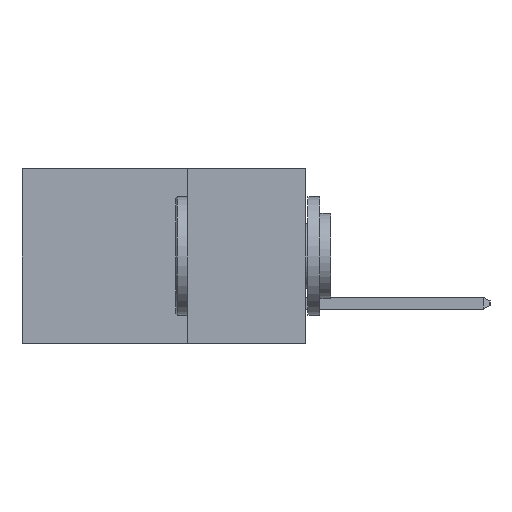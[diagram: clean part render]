
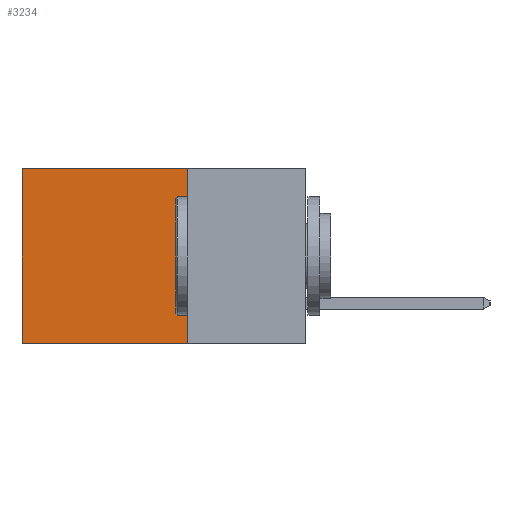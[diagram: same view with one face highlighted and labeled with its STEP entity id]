
A CAD part, left-side view. The second image highlights one B-rep face of the part: STEP entity #3234.
In plain terms, the highlighted planar face has unit normal (-1, 0, 0).
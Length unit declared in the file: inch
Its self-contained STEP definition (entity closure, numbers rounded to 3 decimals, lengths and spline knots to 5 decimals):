
#453 = VECTOR ( 'NONE', #2113, 39.37008 ) ;
#624 = CARTESIAN_POINT ( 'NONE',  ( 0.2615, 0.6, -0.37 ) ) ;
#630 = CARTESIAN_POINT ( 'NONE',  ( 0.2615, 0.25, 0. ) ) ;
#774 = CARTESIAN_POINT ( 'NONE',  ( 0.2615, 0.25, -0.37 ) ) ;
#1173 = EDGE_LOOP ( 'NONE', ( #9363, #12751, #15574, #9798 ) ) ;
#2059 = CARTESIAN_POINT ( 'NONE',  ( 0.2615, 0.25, -0.37 ) ) ;
#2113 = DIRECTION ( 'NONE',  ( 0., 0., -1. ) ) ;
#2167 = AXIS2_PLACEMENT_3D ( 'NONE', #13113, #12889, #12871 ) ;
#3066 = CARTESIAN_POINT ( 'NONE',  ( 0.2615, 0.25, -0.37 ) ) ;
#3168 = CARTESIAN_POINT ( 'NONE',  ( 0.2615, 0.6, 0. ) ) ;
#3234 = ADVANCED_FACE ( 'NONE', ( #12337 ), #14115, .F. ) ;
#3305 = DIRECTION ( 'NONE',  ( 0., 1., 0. ) ) ;
#3522 = VERTEX_POINT ( 'NONE', #3168 ) ;
#4558 = LINE ( 'NONE', #9187, #10623 ) ;
#4650 = VECTOR ( 'NONE', #10969, 39.37008 ) ;
#7011 = LINE ( 'NONE', #774, #453 ) ;
#8507 = VERTEX_POINT ( 'NONE', #630 ) ;
#8822 = EDGE_CURVE ( 'NONE', #8507, #9988, #7011, .T. ) ;
#9187 = CARTESIAN_POINT ( 'NONE',  ( 0.2615, 0.6, -0.37 ) ) ;
#9363 = ORIENTED_EDGE ( 'NONE', *, *, #13162, .T. ) ;
#9756 = CARTESIAN_POINT ( 'NONE',  ( 0.2615, 0.25, 0. ) ) ;
#9798 = ORIENTED_EDGE ( 'NONE', *, *, #10874, .T. ) ;
#9988 = VERTEX_POINT ( 'NONE', #3066 ) ;
#9999 = VERTEX_POINT ( 'NONE', #624 ) ;
#10389 = DIRECTION ( 'NONE',  ( 0., 0., -1. ) ) ;
#10623 = VECTOR ( 'NONE', #10389, 39.37008 ) ;
#10874 = EDGE_CURVE ( 'NONE', #8507, #3522, #11075, .T. ) ;
#10969 = DIRECTION ( 'NONE',  ( 0., 1., 0. ) ) ;
#11075 = LINE ( 'NONE', #9756, #4650 ) ;
#12282 = LINE ( 'NONE', #2059, #12648 ) ;
#12337 = FACE_OUTER_BOUND ( 'NONE', #1173, .T. ) ;
#12648 = VECTOR ( 'NONE', #3305, 39.37008 ) ;
#12751 = ORIENTED_EDGE ( 'NONE', *, *, #13276, .F. ) ;
#12871 = DIRECTION ( 'NONE',  ( 0., 0., -1. ) ) ;
#12889 = DIRECTION ( 'NONE',  ( 1., 0., 0. ) ) ;
#13113 = CARTESIAN_POINT ( 'NONE',  ( 0.2615, 0.25, -0.37 ) ) ;
#13162 = EDGE_CURVE ( 'NONE', #3522, #9999, #4558, .T. ) ;
#13276 = EDGE_CURVE ( 'NONE', #9988, #9999, #12282, .T. ) ;
#14115 = PLANE ( 'NONE',  #2167 ) ;
#15574 = ORIENTED_EDGE ( 'NONE', *, *, #8822, .F. ) ;
